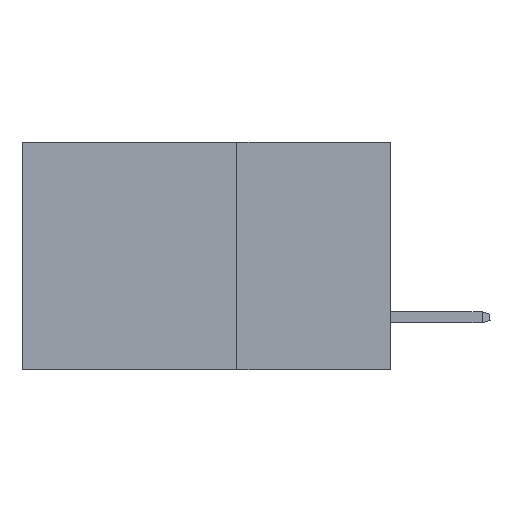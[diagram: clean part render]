
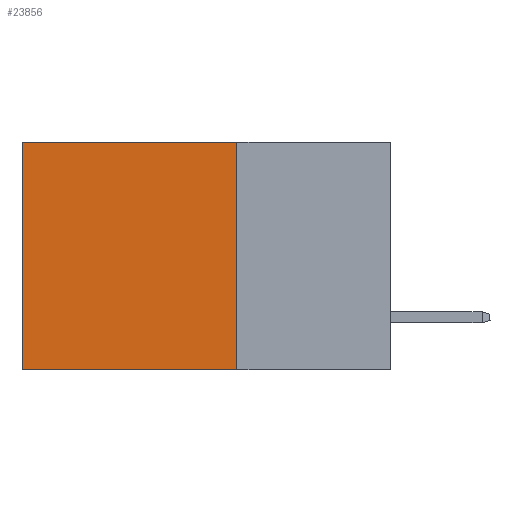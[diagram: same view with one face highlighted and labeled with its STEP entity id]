
A CAD part, left-side view. The second image highlights one B-rep face of the part: STEP entity #23856.
In plain terms, the highlighted planar face has unit normal (-1, 0, 0).
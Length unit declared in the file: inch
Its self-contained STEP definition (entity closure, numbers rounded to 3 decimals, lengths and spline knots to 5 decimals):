
#676 = DIRECTION ( 'NONE',  ( 0., 0., -1. ) ) ;
#790 = EDGE_CURVE ( 'NONE', #1554, #9400, #15025, .T. ) ;
#1554 = VERTEX_POINT ( 'NONE', #14544 ) ;
#2170 = DIRECTION ( 'NONE',  ( 1., 0., 0. ) ) ;
#3758 = LINE ( 'NONE', #9865, #18963 ) ;
#4298 = DIRECTION ( 'NONE',  ( 0., 1., 0. ) ) ;
#5561 = LINE ( 'NONE', #14058, #18723 ) ;
#6842 = AXIS2_PLACEMENT_3D ( 'NONE', #9627, #2170, #19092 ) ;
#7096 = ORIENTED_EDGE ( 'NONE', *, *, #14196, .T. ) ;
#8894 = FACE_OUTER_BOUND ( 'NONE', #20600, .T. ) ;
#9148 = EDGE_CURVE ( 'NONE', #22226, #17634, #15577, .T. ) ;
#9400 = VERTEX_POINT ( 'NONE', #22950 ) ;
#9627 = CARTESIAN_POINT ( 'NONE',  ( 0.2875, 0.25, 0. ) ) ;
#9687 = CARTESIAN_POINT ( 'NONE',  ( 0.2875, 0.25, 0. ) ) ;
#9865 = CARTESIAN_POINT ( 'NONE',  ( 0.2875, 0.25, -0.37 ) ) ;
#11406 = PLANE ( 'NONE',  #6842 ) ;
#12344 = ORIENTED_EDGE ( 'NONE', *, *, #790, .T. ) ;
#12834 = DIRECTION ( 'NONE',  ( 0., 1., 0. ) ) ;
#12909 = DIRECTION ( 'NONE',  ( 0., 0., -1. ) ) ;
#13406 = ORIENTED_EDGE ( 'NONE', *, *, #21702, .F. ) ;
#14058 = CARTESIAN_POINT ( 'NONE',  ( 0.2875, 0.25, 0. ) ) ;
#14196 = EDGE_CURVE ( 'NONE', #22226, #1554, #5561, .T. ) ;
#14544 = CARTESIAN_POINT ( 'NONE',  ( 0.2875, 0.6, 0. ) ) ;
#15025 = LINE ( 'NONE', #23808, #16796 ) ;
#15577 = LINE ( 'NONE', #9687, #19692 ) ;
#16796 = VECTOR ( 'NONE', #12909, 39.37008 ) ;
#16915 = ORIENTED_EDGE ( 'NONE', *, *, #9148, .F. ) ;
#17112 = CARTESIAN_POINT ( 'NONE',  ( 0.2875, 0.25, 0. ) ) ;
#17634 = VERTEX_POINT ( 'NONE', #21996 ) ;
#18723 = VECTOR ( 'NONE', #12834, 39.37008 ) ;
#18963 = VECTOR ( 'NONE', #4298, 39.37008 ) ;
#19092 = DIRECTION ( 'NONE',  ( 0., 0., -1. ) ) ;
#19692 = VECTOR ( 'NONE', #676, 39.37008 ) ;
#20600 = EDGE_LOOP ( 'NONE', ( #12344, #13406, #16915, #7096 ) ) ;
#21702 = EDGE_CURVE ( 'NONE', #17634, #9400, #3758, .T. ) ;
#21996 = CARTESIAN_POINT ( 'NONE',  ( 0.2875, 0.25, -0.37 ) ) ;
#22226 = VERTEX_POINT ( 'NONE', #17112 ) ;
#22950 = CARTESIAN_POINT ( 'NONE',  ( 0.2875, 0.6, -0.37 ) ) ;
#23808 = CARTESIAN_POINT ( 'NONE',  ( 0.2875, 0.6, 0. ) ) ;
#23856 = ADVANCED_FACE ( 'NONE', ( #8894 ), #11406, .F. ) ;
